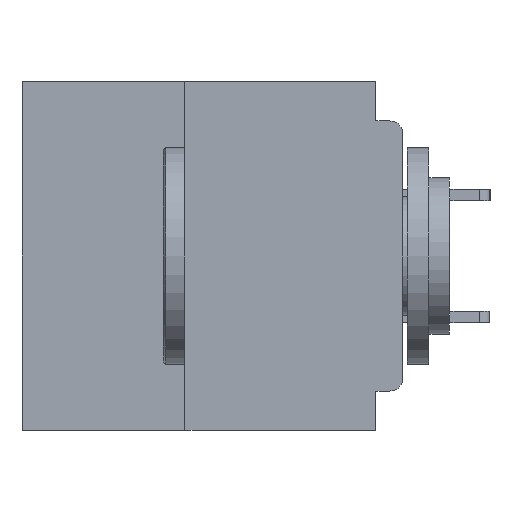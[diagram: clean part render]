
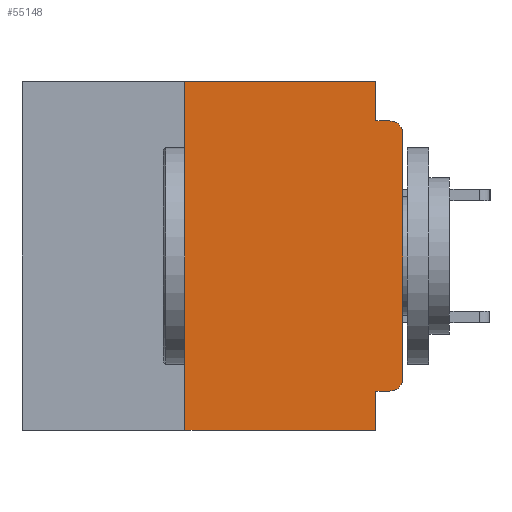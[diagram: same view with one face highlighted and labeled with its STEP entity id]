
A CAD part, left-side view. The second image highlights one B-rep face of the part: STEP entity #55148.
In plain terms, the highlighted planar face has unit normal (-1, 0, 0).
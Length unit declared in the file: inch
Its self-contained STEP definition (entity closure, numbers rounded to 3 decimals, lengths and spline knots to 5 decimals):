
#809 = ORIENTED_EDGE ( 'NONE', *, *, #36239, .T. ) ;
#1007 = VERTEX_POINT ( 'NONE', #39849 ) ;
#2857 = VERTEX_POINT ( 'NONE', #6299 ) ;
#3199 = LINE ( 'NONE', #62423, #53981 ) ;
#3606 = VERTEX_POINT ( 'NONE', #56110 ) ;
#4393 = VECTOR ( 'NONE', #37603, 39.37008 ) ;
#6040 = LINE ( 'NONE', #55288, #52173 ) ;
#6282 = CARTESIAN_POINT ( 'NONE',  ( 0., 0., -0.355 ) ) ;
#6299 = CARTESIAN_POINT ( 'NONE',  ( 0., 0.015, -0.045 ) ) ;
#8450 = CARTESIAN_POINT ( 'NONE',  ( 0., 0.437, 0. ) ) ;
#9271 = EDGE_CURVE ( 'NONE', #3606, #61143, #52734, .T. ) ;
#9644 = EDGE_CURVE ( 'NONE', #60785, #1007, #60350, .T. ) ;
#10096 = CARTESIAN_POINT ( 'NONE',  ( 0., 0.031, -0.045 ) ) ;
#10231 = ORIENTED_EDGE ( 'NONE', *, *, #27063, .T. ) ;
#12015 = EDGE_LOOP ( 'NONE', ( #809, #61206, #62442, #29876, #24352, #44250, #27668, #32362, #47009, #10231 ) ) ;
#13481 = DIRECTION ( 'NONE',  ( 0., 0., -1. ) ) ;
#14754 = VERTEX_POINT ( 'NONE', #16227 ) ;
#16151 = LINE ( 'NONE', #63657, #42300 ) ;
#16227 = CARTESIAN_POINT ( 'NONE',  ( 0., 0.031, -0.355 ) ) ;
#17457 = CARTESIAN_POINT ( 'NONE',  ( 0., 0.437, 0. ) ) ;
#18030 = CARTESIAN_POINT ( 'NONE',  ( 0., 0., 0. ) ) ;
#19146 = EDGE_CURVE ( 'NONE', #34937, #14754, #53642, .T. ) ;
#21339 = VECTOR ( 'NONE', #27422, 39.37008 ) ;
#22663 = VERTEX_POINT ( 'NONE', #10096 ) ;
#24352 = ORIENTED_EDGE ( 'NONE', *, *, #9644, .F. ) ;
#24439 = CARTESIAN_POINT ( 'NONE',  ( 0., 0.015, -0.06 ) ) ;
#24849 = CARTESIAN_POINT ( 'NONE',  ( 0., 0.031, -0.4 ) ) ;
#27063 = EDGE_CURVE ( 'NONE', #34937, #29572, #59187, .T. ) ;
#27422 = DIRECTION ( 'NONE',  ( 0., -1., 0. ) ) ;
#27668 = ORIENTED_EDGE ( 'NONE', *, *, #9271, .T. ) ;
#28219 = PLANE ( 'NONE',  #56713 ) ;
#28322 = DIRECTION ( 'NONE',  ( -1., 0., 0. ) ) ;
#29363 = DIRECTION ( 'NONE',  ( 0., 0., -1. ) ) ;
#29572 = VERTEX_POINT ( 'NONE', #41001 ) ;
#29876 = ORIENTED_EDGE ( 'NONE', *, *, #45764, .F. ) ;
#32169 = CIRCLE ( 'NONE', #55687, 0.015 ) ;
#32362 = ORIENTED_EDGE ( 'NONE', *, *, #59186, .F. ) ;
#32920 = AXIS2_PLACEMENT_3D ( 'NONE', #57522, #28322, #62440 ) ;
#33246 = DIRECTION ( 'NONE',  ( 0., 0., -1. ) ) ;
#34500 = DIRECTION ( 'NONE',  ( 0., 0., 1. ) ) ;
#34937 = VERTEX_POINT ( 'NONE', #41441 ) ;
#36239 = EDGE_CURVE ( 'NONE', #29572, #50227, #55113, .T. ) ;
#36794 = DIRECTION ( 'NONE',  ( 0., -1., 0. ) ) ;
#37019 = EDGE_CURVE ( 'NONE', #50227, #2857, #32169, .T. ) ;
#37603 = DIRECTION ( 'NONE',  ( 0., 0., 1. ) ) ;
#38202 = LINE ( 'NONE', #61063, #62603 ) ;
#39846 = VECTOR ( 'NONE', #54084, 39.37008 ) ;
#39849 = CARTESIAN_POINT ( 'NONE',  ( 0., 0.031, 0. ) ) ;
#40712 = VECTOR ( 'NONE', #59971, 39.37008 ) ;
#41001 = CARTESIAN_POINT ( 'NONE',  ( 0., 0., -0.34 ) ) ;
#41441 = CARTESIAN_POINT ( 'NONE',  ( 0., 0.015, -0.355 ) ) ;
#42300 = VECTOR ( 'NONE', #34500, 39.37008 ) ;
#42945 = DIRECTION ( 'NONE',  ( 1., 0., 0. ) ) ;
#44250 = ORIENTED_EDGE ( 'NONE', *, *, #52818, .F. ) ;
#44543 = CARTESIAN_POINT ( 'NONE',  ( 0., 0.437, -0.4 ) ) ;
#45764 = EDGE_CURVE ( 'NONE', #1007, #22663, #6040, .T. ) ;
#46439 = CARTESIAN_POINT ( 'NONE',  ( 0., 0.25, 0. ) ) ;
#47009 = ORIENTED_EDGE ( 'NONE', *, *, #19146, .F. ) ;
#50227 = VERTEX_POINT ( 'NONE', #51089 ) ;
#51089 = CARTESIAN_POINT ( 'NONE',  ( 0., 0., -0.06 ) ) ;
#51864 = FACE_OUTER_BOUND ( 'NONE', #12015, .T. ) ;
#52173 = VECTOR ( 'NONE', #60212, 39.37008 ) ;
#52734 = LINE ( 'NONE', #44543, #39846 ) ;
#52818 = EDGE_CURVE ( 'NONE', #3606, #60785, #16151, .T. ) ;
#53642 = LINE ( 'NONE', #6282, #40712 ) ;
#53981 = VECTOR ( 'NONE', #33246, 39.37008 ) ;
#54084 = DIRECTION ( 'NONE',  ( 0., -1., 0. ) ) ;
#55006 = EDGE_CURVE ( 'NONE', #22663, #2857, #38202, .T. ) ;
#55113 = LINE ( 'NONE', #18030, #4393 ) ;
#55148 = ADVANCED_FACE ( 'NONE', ( #51864 ), #28219, .F. ) ;
#55288 = CARTESIAN_POINT ( 'NONE',  ( 0., 0.031, 0. ) ) ;
#55687 = AXIS2_PLACEMENT_3D ( 'NONE', #24439, #58591, #29363 ) ;
#56110 = CARTESIAN_POINT ( 'NONE',  ( 0., 0.25, -0.4 ) ) ;
#56713 = AXIS2_PLACEMENT_3D ( 'NONE', #8450, #42945, #13481 ) ;
#57522 = CARTESIAN_POINT ( 'NONE',  ( 0., 0.015, -0.34 ) ) ;
#58591 = DIRECTION ( 'NONE',  ( -1., 0., 0. ) ) ;
#59186 = EDGE_CURVE ( 'NONE', #14754, #61143, #3199, .T. ) ;
#59187 = CIRCLE ( 'NONE', #32920, 0.015 ) ;
#59971 = DIRECTION ( 'NONE',  ( 0., 1., 0. ) ) ;
#60212 = DIRECTION ( 'NONE',  ( 0., 0., -1. ) ) ;
#60350 = LINE ( 'NONE', #17457, #21339 ) ;
#60785 = VERTEX_POINT ( 'NONE', #46439 ) ;
#61063 = CARTESIAN_POINT ( 'NONE',  ( 0., 0., -0.045 ) ) ;
#61143 = VERTEX_POINT ( 'NONE', #24849 ) ;
#61206 = ORIENTED_EDGE ( 'NONE', *, *, #37019, .T. ) ;
#62423 = CARTESIAN_POINT ( 'NONE',  ( 0., 0.031, -0.4 ) ) ;
#62440 = DIRECTION ( 'NONE',  ( 0., 0., -1. ) ) ;
#62442 = ORIENTED_EDGE ( 'NONE', *, *, #55006, .F. ) ;
#62603 = VECTOR ( 'NONE', #36794, 39.37008 ) ;
#63657 = CARTESIAN_POINT ( 'NONE',  ( 0., 0.25, -0.4 ) ) ;
